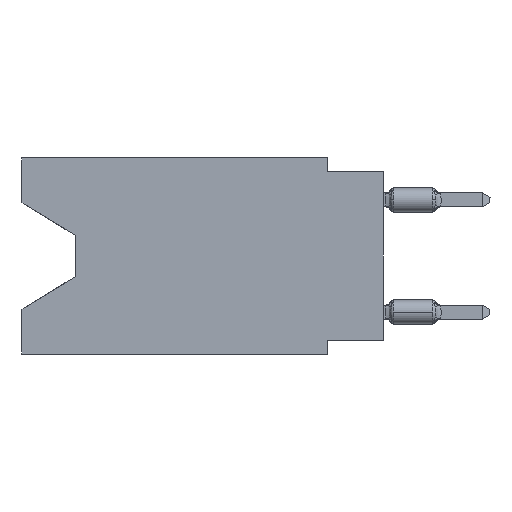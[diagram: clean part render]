
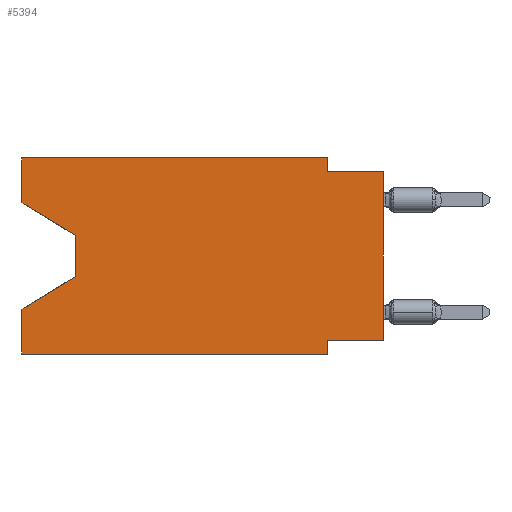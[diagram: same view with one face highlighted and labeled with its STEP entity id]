
A CAD part, left-side view. The second image highlights one B-rep face of the part: STEP entity #5394.
In plain terms, the highlighted planar face has unit normal (-1, 0, 0).
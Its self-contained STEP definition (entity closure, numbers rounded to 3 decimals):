
#498 = CARTESIAN_POINT ( 'NONE',  ( 0., 0., -8.255 ) ) ;
#715 = LINE ( 'NONE', #45746, #55850 ) ;
#1367 = DIRECTION ( 'NONE',  ( 0., 0., 1. ) ) ;
#1900 = CARTESIAN_POINT ( 'NONE',  ( 0., 0., -0.635 ) ) ;
#3200 = CARTESIAN_POINT ( 'NONE',  ( 0., 2.54, -8.255 ) ) ;
#4154 = EDGE_CURVE ( 'NONE', #22663, #52151, #50760, .T. ) ;
#4649 = CARTESIAN_POINT ( 'NONE',  ( 0., 16.383, 0. ) ) ;
#5394 = ADVANCED_FACE ( 'NONE', ( #10642 ), #5414, .F. ) ;
#5414 = PLANE ( 'NONE',  #49639 ) ;
#5898 = EDGE_CURVE ( 'NONE', #8397, #62694, #47408, .T. ) ;
#7244 = VECTOR ( 'NONE', #24204, 1000. ) ;
#8081 = VERTEX_POINT ( 'NONE', #32426 ) ;
#8397 = VERTEX_POINT ( 'NONE', #60101 ) ;
#9001 = CARTESIAN_POINT ( 'NONE',  ( 0., 0., 0. ) ) ;
#9589 = EDGE_CURVE ( 'NONE', #52151, #34914, #28927, .T. ) ;
#9825 = CARTESIAN_POINT ( 'NONE',  ( 0., 16.383, -8.89 ) ) ;
#10626 = DIRECTION ( 'NONE',  ( 0., 1., 0. ) ) ;
#10642 = FACE_OUTER_BOUND ( 'NONE', #34459, .T. ) ;
#10656 = VECTOR ( 'NONE', #14025, 1000. ) ;
#10870 = CARTESIAN_POINT ( 'NONE',  ( 0., 16.383, 0. ) ) ;
#11461 = DIRECTION ( 'NONE',  ( 0., 0., -1. ) ) ;
#11947 = ORIENTED_EDGE ( 'NONE', *, *, #19719, .T. ) ;
#12737 = DIRECTION ( 'NONE',  ( 0., 0., 1. ) ) ;
#13211 = VECTOR ( 'NONE', #14854, 1000. ) ;
#13283 = CARTESIAN_POINT ( 'NONE',  ( 0., 13.97, -5.385 ) ) ;
#13879 = ORIENTED_EDGE ( 'NONE', *, *, #51948, .F. ) ;
#14025 = DIRECTION ( 'NONE',  ( 0., 0.855, -0.519 ) ) ;
#14723 = CARTESIAN_POINT ( 'NONE',  ( 0., 2.54, -0.635 ) ) ;
#14854 = DIRECTION ( 'NONE',  ( 0., 0., 1. ) ) ;
#15317 = ORIENTED_EDGE ( 'NONE', *, *, #55475, .F. ) ;
#17067 = EDGE_CURVE ( 'NONE', #46753, #34914, #29429, .T. ) ;
#19561 = EDGE_CURVE ( 'NONE', #28369, #50391, #55592, .T. ) ;
#19655 = VECTOR ( 'NONE', #54691, 1000. ) ;
#19719 = EDGE_CURVE ( 'NONE', #62694, #48016, #23168, .T. ) ;
#20799 = CARTESIAN_POINT ( 'NONE',  ( 0., 2.54, 0. ) ) ;
#21975 = ORIENTED_EDGE ( 'NONE', *, *, #57064, .T. ) ;
#22663 = VERTEX_POINT ( 'NONE', #55926 ) ;
#22822 = ORIENTED_EDGE ( 'NONE', *, *, #17067, .T. ) ;
#22907 = CARTESIAN_POINT ( 'NONE',  ( 0., 16.383, -2.038 ) ) ;
#23168 = LINE ( 'NONE', #33628, #10656 ) ;
#24204 = DIRECTION ( 'NONE',  ( 0., -1., 0. ) ) ;
#24681 = CARTESIAN_POINT ( 'NONE',  ( 0., 16.383, 0. ) ) ;
#26885 = CARTESIAN_POINT ( 'NONE',  ( 0., 16.383, -2.038 ) ) ;
#28369 = VERTEX_POINT ( 'NONE', #26885 ) ;
#28909 = VECTOR ( 'NONE', #47080, 1000. ) ;
#28927 = LINE ( 'NONE', #54021, #30390 ) ;
#29429 = LINE ( 'NONE', #9825, #7244 ) ;
#29592 = LINE ( 'NONE', #24681, #19655 ) ;
#30390 = VECTOR ( 'NONE', #11461, 1000. ) ;
#31074 = ORIENTED_EDGE ( 'NONE', *, *, #33714, .F. ) ;
#31757 = ORIENTED_EDGE ( 'NONE', *, *, #5898, .T. ) ;
#31967 = LINE ( 'NONE', #1900, #39303 ) ;
#32426 = CARTESIAN_POINT ( 'NONE',  ( 0., 0., -0.635 ) ) ;
#33628 = CARTESIAN_POINT ( 'NONE',  ( 0., 13.97, -5.385 ) ) ;
#33714 = EDGE_CURVE ( 'NONE', #46753, #48016, #715, .T. ) ;
#34140 = LINE ( 'NONE', #9001, #13211 ) ;
#34286 = VECTOR ( 'NONE', #41689, 1000. ) ;
#34459 = EDGE_LOOP ( 'NONE', ( #37085, #31757, #11947, #31074, #22822, #44349, #61244, #21975, #13879, #15317, #34949, #55949 ) ) ;
#34510 = VERTEX_POINT ( 'NONE', #14723 ) ;
#34914 = VERTEX_POINT ( 'NONE', #50446 ) ;
#34949 = ORIENTED_EDGE ( 'NONE', *, *, #52619, .F. ) ;
#37085 = ORIENTED_EDGE ( 'NONE', *, *, #53385, .T. ) ;
#39303 = VECTOR ( 'NONE', #62292, 1000. ) ;
#40075 = CARTESIAN_POINT ( 'NONE',  ( 0., 16.383, -6.852 ) ) ;
#41689 = DIRECTION ( 'NONE',  ( 0., 0., -1. ) ) ;
#44349 = ORIENTED_EDGE ( 'NONE', *, *, #9589, .F. ) ;
#44920 = DIRECTION ( 'NONE',  ( 0., 0., -1. ) ) ;
#45746 = CARTESIAN_POINT ( 'NONE',  ( 0., 16.383, 0. ) ) ;
#46753 = VERTEX_POINT ( 'NONE', #54752 ) ;
#47080 = DIRECTION ( 'NONE',  ( 0., 0., -1. ) ) ;
#47408 = LINE ( 'NONE', #62440, #28909 ) ;
#48016 = VERTEX_POINT ( 'NONE', #40075 ) ;
#49639 = AXIS2_PLACEMENT_3D ( 'NONE', #49815, #54727, #44920 ) ;
#49815 = CARTESIAN_POINT ( 'NONE',  ( 0., 16.383, 0. ) ) ;
#50391 = VERTEX_POINT ( 'NONE', #4649 ) ;
#50446 = CARTESIAN_POINT ( 'NONE',  ( 0., 2.54, -8.89 ) ) ;
#50760 = LINE ( 'NONE', #498, #52827 ) ;
#51490 = LINE ( 'NONE', #57366, #34286 ) ;
#51948 = EDGE_CURVE ( 'NONE', #34510, #8081, #31967, .T. ) ;
#52151 = VERTEX_POINT ( 'NONE', #3200 ) ;
#52603 = DIRECTION ( 'NONE',  ( 0., -0.855, -0.519 ) ) ;
#52619 = EDGE_CURVE ( 'NONE', #50391, #61326, #29592, .T. ) ;
#52827 = VECTOR ( 'NONE', #10626, 1000. ) ;
#53385 = EDGE_CURVE ( 'NONE', #28369, #8397, #56540, .T. ) ;
#54021 = CARTESIAN_POINT ( 'NONE',  ( 0., 2.54, -8.89 ) ) ;
#54691 = DIRECTION ( 'NONE',  ( 0., -1., 0. ) ) ;
#54727 = DIRECTION ( 'NONE',  ( 1., 0., 0. ) ) ;
#54752 = CARTESIAN_POINT ( 'NONE',  ( 0., 16.383, -8.89 ) ) ;
#55475 = EDGE_CURVE ( 'NONE', #61326, #34510, #51490, .T. ) ;
#55592 = LINE ( 'NONE', #10870, #56511 ) ;
#55850 = VECTOR ( 'NONE', #1367, 1000. ) ;
#55926 = CARTESIAN_POINT ( 'NONE',  ( 0., 0., -8.255 ) ) ;
#55949 = ORIENTED_EDGE ( 'NONE', *, *, #19561, .F. ) ;
#56511 = VECTOR ( 'NONE', #12737, 1000. ) ;
#56540 = LINE ( 'NONE', #22907, #61342 ) ;
#57064 = EDGE_CURVE ( 'NONE', #22663, #8081, #34140, .T. ) ;
#57366 = CARTESIAN_POINT ( 'NONE',  ( 0., 2.54, 0. ) ) ;
#60101 = CARTESIAN_POINT ( 'NONE',  ( 0., 13.97, -3.505 ) ) ;
#61244 = ORIENTED_EDGE ( 'NONE', *, *, #4154, .F. ) ;
#61326 = VERTEX_POINT ( 'NONE', #20799 ) ;
#61342 = VECTOR ( 'NONE', #52603, 1000. ) ;
#62292 = DIRECTION ( 'NONE',  ( 0., -1., 0. ) ) ;
#62440 = CARTESIAN_POINT ( 'NONE',  ( 0., 13.97, -3.505 ) ) ;
#62694 = VERTEX_POINT ( 'NONE', #13283 ) ;
